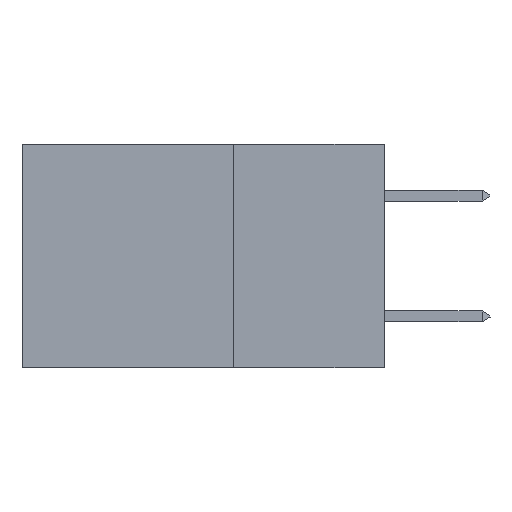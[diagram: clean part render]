
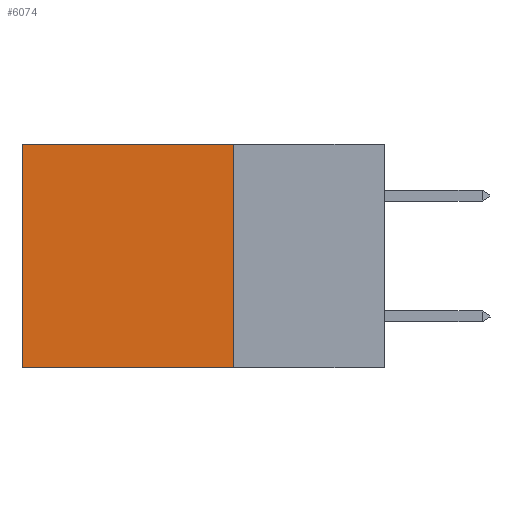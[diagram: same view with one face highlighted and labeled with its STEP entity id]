
A CAD part, left-side view. The second image highlights one B-rep face of the part: STEP entity #6074.
In plain terms, the highlighted planar face has unit normal (-1, 0, 0).
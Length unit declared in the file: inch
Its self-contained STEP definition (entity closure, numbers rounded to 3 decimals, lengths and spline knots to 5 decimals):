
#952 = CARTESIAN_POINT ( 'NONE',  ( 0.2875, 0.6, 0. ) ) ;
#1526 = CARTESIAN_POINT ( 'NONE',  ( 0.2875, 0.25, 0. ) ) ;
#3425 = EDGE_LOOP ( 'NONE', ( #26281, #9071, #5929, #8572 ) ) ;
#4309 = VECTOR ( 'NONE', #5722, 39.37008 ) ;
#4512 = DIRECTION ( 'NONE',  ( 1., 0., 0. ) ) ;
#4776 = DIRECTION ( 'NONE',  ( 0., 1., 0. ) ) ;
#5368 = VECTOR ( 'NONE', #14056, 39.37008 ) ;
#5572 = VECTOR ( 'NONE', #10010, 39.37008 ) ;
#5722 = DIRECTION ( 'NONE',  ( 0., 0., -1. ) ) ;
#5929 = ORIENTED_EDGE ( 'NONE', *, *, #12328, .F. ) ;
#5955 = LINE ( 'NONE', #27602, #8081 ) ;
#6074 = ADVANCED_FACE ( 'NONE', ( #25874 ), #15302, .F. ) ;
#6605 = LINE ( 'NONE', #28656, #5572 ) ;
#7755 = VERTEX_POINT ( 'NONE', #19918 ) ;
#8081 = VECTOR ( 'NONE', #4776, 39.37008 ) ;
#8572 = ORIENTED_EDGE ( 'NONE', *, *, #8897, .T. ) ;
#8897 = EDGE_CURVE ( 'NONE', #7755, #24286, #5955, .T. ) ;
#9071 = ORIENTED_EDGE ( 'NONE', *, *, #15004, .F. ) ;
#9623 = CARTESIAN_POINT ( 'NONE',  ( 0.2875, 0.25, -0.37 ) ) ;
#10010 = DIRECTION ( 'NONE',  ( 0., 1., 0. ) ) ;
#10168 = CARTESIAN_POINT ( 'NONE',  ( 0.2875, 0.6, -0.37 ) ) ;
#11458 = LINE ( 'NONE', #16693, #5368 ) ;
#12328 = EDGE_CURVE ( 'NONE', #7755, #24998, #11458, .T. ) ;
#14056 = DIRECTION ( 'NONE',  ( 0., 0., -1. ) ) ;
#15004 = EDGE_CURVE ( 'NONE', #24998, #15814, #6605, .T. ) ;
#15302 = PLANE ( 'NONE',  #15983 ) ;
#15814 = VERTEX_POINT ( 'NONE', #10168 ) ;
#15983 = AXIS2_PLACEMENT_3D ( 'NONE', #1526, #4512, #26266 ) ;
#16693 = CARTESIAN_POINT ( 'NONE',  ( 0.2875, 0.25, 0. ) ) ;
#18940 = CARTESIAN_POINT ( 'NONE',  ( 0.2875, 0.6, 0. ) ) ;
#19918 = CARTESIAN_POINT ( 'NONE',  ( 0.2875, 0.25, 0. ) ) ;
#24286 = VERTEX_POINT ( 'NONE', #18940 ) ;
#24998 = VERTEX_POINT ( 'NONE', #9623 ) ;
#25874 = FACE_OUTER_BOUND ( 'NONE', #3425, .T. ) ;
#26266 = DIRECTION ( 'NONE',  ( 0., 0., -1. ) ) ;
#26281 = ORIENTED_EDGE ( 'NONE', *, *, #28340, .T. ) ;
#26297 = LINE ( 'NONE', #952, #4309 ) ;
#27602 = CARTESIAN_POINT ( 'NONE',  ( 0.2875, 0.25, 0. ) ) ;
#28340 = EDGE_CURVE ( 'NONE', #24286, #15814, #26297, .T. ) ;
#28656 = CARTESIAN_POINT ( 'NONE',  ( 0.2875, 0.25, -0.37 ) ) ;
